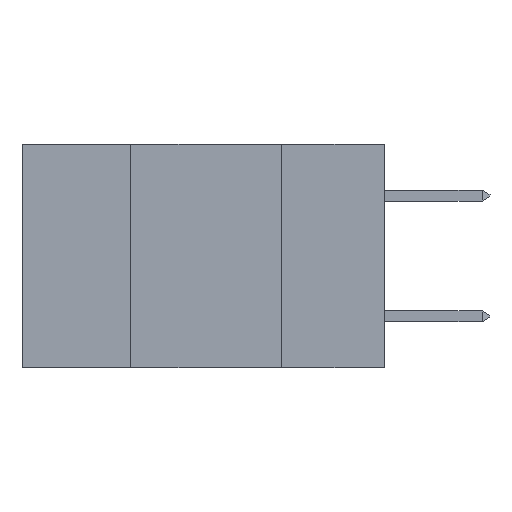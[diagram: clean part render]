
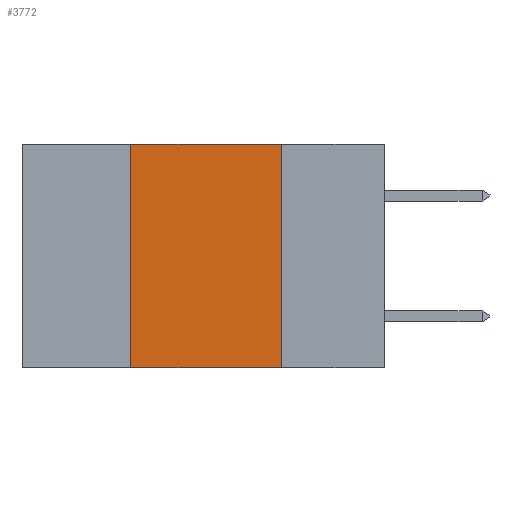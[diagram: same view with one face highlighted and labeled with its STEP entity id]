
A CAD part, left-side view. The second image highlights one B-rep face of the part: STEP entity #3772.
In plain terms, the highlighted planar face has unit normal (-1, 0, 0).
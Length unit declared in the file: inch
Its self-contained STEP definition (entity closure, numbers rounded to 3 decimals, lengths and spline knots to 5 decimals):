
#2315 = CARTESIAN_POINT ( 'NONE',  ( 0., 0.6, -0.37 ) ) ;
#2810 = ORIENTED_EDGE ( 'NONE', *, *, #9701, .F. ) ;
#3054 = DIRECTION ( 'NONE',  ( 0., 0., -1. ) ) ;
#3702 = VECTOR ( 'NONE', #12656, 39.37008 ) ;
#3772 = ADVANCED_FACE ( 'NONE', ( #4145 ), #5084, .F. ) ;
#4145 = FACE_OUTER_BOUND ( 'NONE', #12767, .T. ) ;
#4291 = LINE ( 'NONE', #15005, #12344 ) ;
#5084 = PLANE ( 'NONE',  #13307 ) ;
#5226 = DIRECTION ( 'NONE',  ( 0., 0., -1. ) ) ;
#5637 = DIRECTION ( 'NONE',  ( 1., 0., 0. ) ) ;
#5800 = LINE ( 'NONE', #19340, #9841 ) ;
#5849 = VERTEX_POINT ( 'NONE', #19440 ) ;
#6298 = CARTESIAN_POINT ( 'NONE',  ( 0., 0.42, 0. ) ) ;
#7484 = DIRECTION ( 'NONE',  ( 0., -1., 0. ) ) ;
#7561 = CARTESIAN_POINT ( 'NONE',  ( 0., 0.42, 0. ) ) ;
#8979 = ORIENTED_EDGE ( 'NONE', *, *, #18001, .T. ) ;
#9701 = EDGE_CURVE ( 'NONE', #19500, #20283, #11175, .T. ) ;
#9841 = VECTOR ( 'NONE', #7484, 39.37008 ) ;
#11171 = ORIENTED_EDGE ( 'NONE', *, *, #17579, .F. ) ;
#11175 = LINE ( 'NONE', #7561, #19537 ) ;
#12344 = VECTOR ( 'NONE', #3054, 39.37008 ) ;
#12627 = DIRECTION ( 'NONE',  ( 0., 0., 1. ) ) ;
#12656 = DIRECTION ( 'NONE',  ( 0., -1., 0. ) ) ;
#12767 = EDGE_LOOP ( 'NONE', ( #11171, #18458, #2810, #8979 ) ) ;
#13307 = AXIS2_PLACEMENT_3D ( 'NONE', #18083, #5637, #5226 ) ;
#14221 = EDGE_CURVE ( 'NONE', #20283, #5849, #5800, .T. ) ;
#15005 = CARTESIAN_POINT ( 'NONE',  ( 0., 0.17, 0. ) ) ;
#16766 = CARTESIAN_POINT ( 'NONE',  ( 0., 0.42, -0.37 ) ) ;
#17051 = CARTESIAN_POINT ( 'NONE',  ( 0., 0.17, -0.37 ) ) ;
#17579 = EDGE_CURVE ( 'NONE', #5849, #19634, #4291, .T. ) ;
#17802 = LINE ( 'NONE', #2315, #3702 ) ;
#18001 = EDGE_CURVE ( 'NONE', #19500, #19634, #17802, .T. ) ;
#18083 = CARTESIAN_POINT ( 'NONE',  ( 0., 0.6, 0. ) ) ;
#18458 = ORIENTED_EDGE ( 'NONE', *, *, #14221, .F. ) ;
#19340 = CARTESIAN_POINT ( 'NONE',  ( 0., 0.6, 0. ) ) ;
#19440 = CARTESIAN_POINT ( 'NONE',  ( 0., 0.17, 0. ) ) ;
#19500 = VERTEX_POINT ( 'NONE', #16766 ) ;
#19537 = VECTOR ( 'NONE', #12627, 39.37008 ) ;
#19634 = VERTEX_POINT ( 'NONE', #17051 ) ;
#20283 = VERTEX_POINT ( 'NONE', #6298 ) ;
